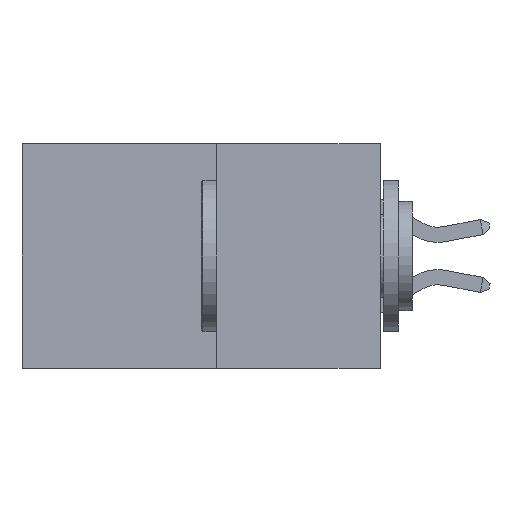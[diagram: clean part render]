
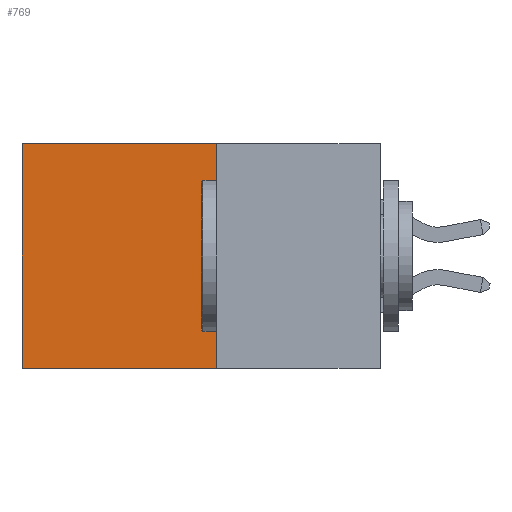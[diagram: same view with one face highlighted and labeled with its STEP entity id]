
A CAD part, left-side view. The second image highlights one B-rep face of the part: STEP entity #769.
In plain terms, the highlighted planar face has unit normal (-1, 0, 0).
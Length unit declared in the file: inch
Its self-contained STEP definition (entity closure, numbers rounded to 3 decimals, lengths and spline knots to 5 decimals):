
#769 = ADVANCED_FACE ( 'NONE', ( #6954 ), #1533, .F. ) ;
#1480 = VERTEX_POINT ( 'NONE', #14237 ) ;
#1533 = PLANE ( 'NONE',  #3346 ) ;
#1809 = LINE ( 'NONE', #8559, #13296 ) ;
#2060 = EDGE_CURVE ( 'NONE', #1480, #6688, #11539, .T. ) ;
#2682 = CARTESIAN_POINT ( 'NONE',  ( 0.277, 0.59, -0.37 ) ) ;
#3056 = DIRECTION ( 'NONE',  ( 0., 1., 0. ) ) ;
#3346 = AXIS2_PLACEMENT_3D ( 'NONE', #7108, #3907, #6461 ) ;
#3907 = DIRECTION ( 'NONE',  ( 1., 0., 0. ) ) ;
#4087 = CARTESIAN_POINT ( 'NONE',  ( 0.277, 0.59, -0.37 ) ) ;
#4135 = DIRECTION ( 'NONE',  ( 0., 0., -1. ) ) ;
#5073 = DIRECTION ( 'NONE',  ( 0., 1., 0. ) ) ;
#5245 = DIRECTION ( 'NONE',  ( 0., 0., -1. ) ) ;
#5976 = VECTOR ( 'NONE', #3056, 39.37008 ) ;
#6461 = DIRECTION ( 'NONE',  ( 0., 0., -1. ) ) ;
#6688 = VERTEX_POINT ( 'NONE', #7008 ) ;
#6954 = FACE_OUTER_BOUND ( 'NONE', #10386, .T. ) ;
#7008 = CARTESIAN_POINT ( 'NONE',  ( 0.277, 0.59, 0. ) ) ;
#7108 = CARTESIAN_POINT ( 'NONE',  ( 0.277, 0.27, -0.37 ) ) ;
#7174 = ORIENTED_EDGE ( 'NONE', *, *, #12982, .F. ) ;
#7296 = VERTEX_POINT ( 'NONE', #13012 ) ;
#8221 = ORIENTED_EDGE ( 'NONE', *, *, #2060, .T. ) ;
#8559 = CARTESIAN_POINT ( 'NONE',  ( 0.277, 0.27, -0.37 ) ) ;
#8686 = VECTOR ( 'NONE', #5245, 39.37008 ) ;
#9020 = LINE ( 'NONE', #4087, #8686 ) ;
#9565 = ORIENTED_EDGE ( 'NONE', *, *, #10236, .T. ) ;
#9729 = CARTESIAN_POINT ( 'NONE',  ( 0.277, 0.27, -0.37 ) ) ;
#9830 = CARTESIAN_POINT ( 'NONE',  ( 0.277, 0.27, 0. ) ) ;
#10236 = EDGE_CURVE ( 'NONE', #6688, #13072, #9020, .T. ) ;
#10386 = EDGE_LOOP ( 'NONE', ( #9565, #7174, #14352, #8221 ) ) ;
#11539 = LINE ( 'NONE', #9830, #14092 ) ;
#11777 = LINE ( 'NONE', #9729, #5976 ) ;
#12982 = EDGE_CURVE ( 'NONE', #7296, #13072, #11777, .T. ) ;
#13012 = CARTESIAN_POINT ( 'NONE',  ( 0.277, 0.27, -0.37 ) ) ;
#13072 = VERTEX_POINT ( 'NONE', #2682 ) ;
#13296 = VECTOR ( 'NONE', #4135, 39.37008 ) ;
#13957 = EDGE_CURVE ( 'NONE', #1480, #7296, #1809, .T. ) ;
#14092 = VECTOR ( 'NONE', #5073, 39.37008 ) ;
#14237 = CARTESIAN_POINT ( 'NONE',  ( 0.277, 0.27, 0. ) ) ;
#14352 = ORIENTED_EDGE ( 'NONE', *, *, #13957, .F. ) ;
